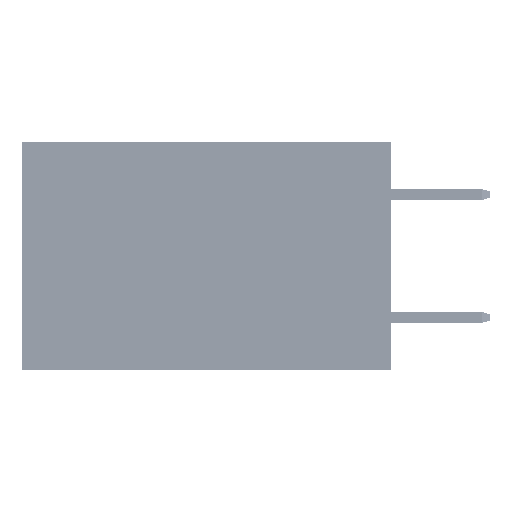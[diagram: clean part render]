
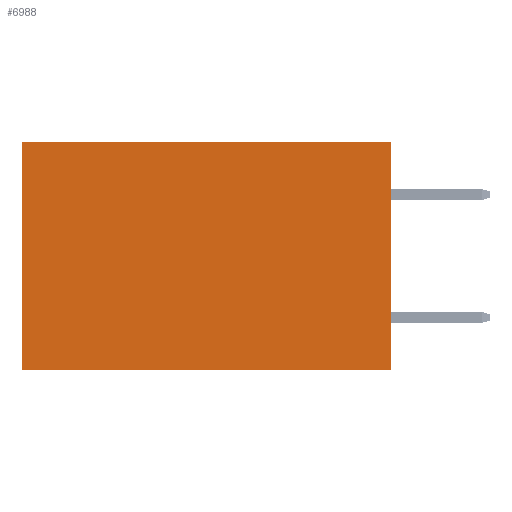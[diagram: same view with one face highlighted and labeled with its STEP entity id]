
A CAD part, left-side view. The second image highlights one B-rep face of the part: STEP entity #6988.
In plain terms, the highlighted planar face has unit normal (-1, 0, 0).
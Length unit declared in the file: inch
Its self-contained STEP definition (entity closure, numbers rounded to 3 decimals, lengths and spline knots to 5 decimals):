
#594 = VERTEX_POINT ( 'NONE', #39962 ) ;
#1682 = EDGE_CURVE ( 'NONE', #594, #50212, #17150, .T. ) ;
#1700 = VECTOR ( 'NONE', #41120, 39.37008 ) ;
#1737 = LINE ( 'NONE', #18299, #32639 ) ;
#6743 = LINE ( 'NONE', #12963, #1700 ) ;
#6988 = ADVANCED_FACE ( 'NONE', ( #40959 ), #13374, .F. ) ;
#11572 = CARTESIAN_POINT ( 'NONE',  ( 0.2875, 0.6, 0. ) ) ;
#12717 = VECTOR ( 'NONE', #42737, 39.37008 ) ;
#12963 = CARTESIAN_POINT ( 'NONE',  ( 0.2875, 0., 0. ) ) ;
#13374 = PLANE ( 'NONE',  #36408 ) ;
#13541 = DIRECTION ( 'NONE',  ( 0., 0., -1. ) ) ;
#13726 = DIRECTION ( 'NONE',  ( 1., 0., 0. ) ) ;
#14152 = EDGE_CURVE ( 'NONE', #49578, #48898, #16505, .T. ) ;
#16505 = LINE ( 'NONE', #18462, #12717 ) ;
#17150 = LINE ( 'NONE', #11572, #26564 ) ;
#18299 = CARTESIAN_POINT ( 'NONE',  ( 0.2875, 0., -0.37 ) ) ;
#18462 = CARTESIAN_POINT ( 'NONE',  ( 0.2875, 0., 0. ) ) ;
#19725 = ORIENTED_EDGE ( 'NONE', *, *, #43574, .F. ) ;
#21313 = CARTESIAN_POINT ( 'NONE',  ( 0.2875, 0., 0. ) ) ;
#23367 = DIRECTION ( 'NONE',  ( 0., 0., -1. ) ) ;
#26374 = DIRECTION ( 'NONE',  ( 0., 1., 0. ) ) ;
#26564 = VECTOR ( 'NONE', #23367, 39.37008 ) ;
#28571 = CARTESIAN_POINT ( 'NONE',  ( 0.2875, 0., 0. ) ) ;
#31643 = CARTESIAN_POINT ( 'NONE',  ( 0.2875, 0., -0.37 ) ) ;
#32639 = VECTOR ( 'NONE', #26374, 39.37008 ) ;
#36408 = AXIS2_PLACEMENT_3D ( 'NONE', #21313, #13726, #13541 ) ;
#38375 = EDGE_CURVE ( 'NONE', #49578, #594, #6743, .T. ) ;
#39962 = CARTESIAN_POINT ( 'NONE',  ( 0.2875, 0.6, 0. ) ) ;
#40006 = CARTESIAN_POINT ( 'NONE',  ( 0.2875, 0.6, -0.37 ) ) ;
#40959 = FACE_OUTER_BOUND ( 'NONE', #46984, .T. ) ;
#41120 = DIRECTION ( 'NONE',  ( 0., 1., 0. ) ) ;
#42737 = DIRECTION ( 'NONE',  ( 0., 0., -1. ) ) ;
#43574 = EDGE_CURVE ( 'NONE', #48898, #50212, #1737, .T. ) ;
#44022 = ORIENTED_EDGE ( 'NONE', *, *, #14152, .F. ) ;
#45916 = ORIENTED_EDGE ( 'NONE', *, *, #1682, .T. ) ;
#46984 = EDGE_LOOP ( 'NONE', ( #45916, #19725, #44022, #47206 ) ) ;
#47206 = ORIENTED_EDGE ( 'NONE', *, *, #38375, .T. ) ;
#48898 = VERTEX_POINT ( 'NONE', #31643 ) ;
#49578 = VERTEX_POINT ( 'NONE', #28571 ) ;
#50212 = VERTEX_POINT ( 'NONE', #40006 ) ;
